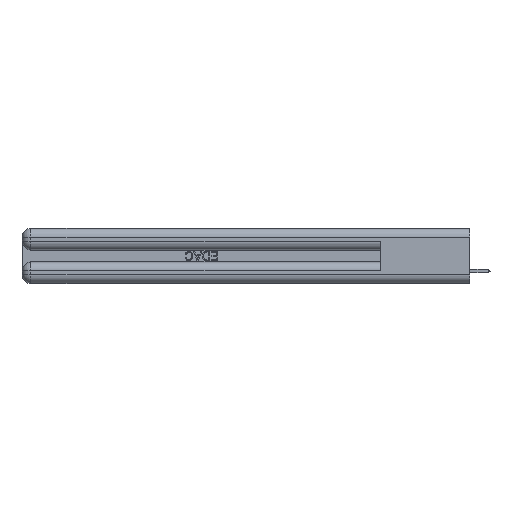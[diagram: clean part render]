
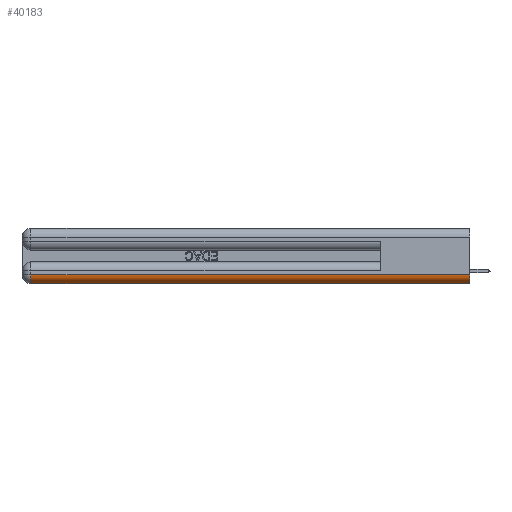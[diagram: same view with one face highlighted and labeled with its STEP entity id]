
A CAD part, left-side view. The second image highlights one B-rep face of the part: STEP entity #40183.
In plain terms, the highlighted cylindrical face has radius 1.524 mm (diameter 3.048 mm), a partial arc.
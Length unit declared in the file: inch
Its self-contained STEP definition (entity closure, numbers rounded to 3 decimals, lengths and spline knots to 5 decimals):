
#938 = DIRECTION ( 'NONE',  ( 0., -1., 0. ) ) ;
#4391 = EDGE_CURVE ( 'NONE', #38778, #20367, #21071, .T. ) ;
#5173 = CARTESIAN_POINT ( 'NONE',  ( 0.06, 0., 0. ) ) ;
#5672 = VECTOR ( 'NONE', #938, 39.37008 ) ;
#6079 = CARTESIAN_POINT ( 'NONE',  ( 0.06, 2.94, 0. ) ) ;
#6116 = LINE ( 'NONE', #17339, #40476 ) ;
#7012 = AXIS2_PLACEMENT_3D ( 'NONE', #14350, #36094, #39672 ) ;
#9419 = DIRECTION ( 'NONE',  ( 0., -1., 0. ) ) ;
#10543 = VERTEX_POINT ( 'NONE', #6079 ) ;
#13378 = EDGE_CURVE ( 'NONE', #28678, #38778, #43937, .T. ) ;
#13647 = ORIENTED_EDGE ( 'NONE', *, *, #13378, .F. ) ;
#14350 = CARTESIAN_POINT ( 'NONE',  ( 0.06, 2.94, 0.06 ) ) ;
#15089 = FACE_OUTER_BOUND ( 'NONE', #19621, .T. ) ;
#17255 = AXIS2_PLACEMENT_3D ( 'NONE', #27853, #9419, #34544 ) ;
#17339 = CARTESIAN_POINT ( 'NONE',  ( 0.06, 3., 0. ) ) ;
#17907 = CYLINDRICAL_SURFACE ( 'NONE', #21600, 0.06 ) ;
#18154 = ORIENTED_EDGE ( 'NONE', *, *, #30021, .F. ) ;
#19589 = CARTESIAN_POINT ( 'NONE',  ( 0., 0., 0.06 ) ) ;
#19608 = CIRCLE ( 'NONE', #7012, 0.06 ) ;
#19621 = EDGE_LOOP ( 'NONE', ( #29744, #13647, #32563, #18154 ) ) ;
#19750 = DIRECTION ( 'NONE',  ( 0., 0., 1. ) ) ;
#20367 = VERTEX_POINT ( 'NONE', #5173 ) ;
#21071 = CIRCLE ( 'NONE', #17255, 0.06 ) ;
#21600 = AXIS2_PLACEMENT_3D ( 'NONE', #34498, #30189, #19750 ) ;
#26704 = CARTESIAN_POINT ( 'NONE',  ( 0., 0., 0.06 ) ) ;
#27853 = CARTESIAN_POINT ( 'NONE',  ( 0.06, 0., 0.06 ) ) ;
#28678 = VERTEX_POINT ( 'NONE', #43455 ) ;
#29744 = ORIENTED_EDGE ( 'NONE', *, *, #4391, .F. ) ;
#30021 = EDGE_CURVE ( 'NONE', #20367, #10543, #6116, .T. ) ;
#30189 = DIRECTION ( 'NONE',  ( 0., 1., 0. ) ) ;
#32563 = ORIENTED_EDGE ( 'NONE', *, *, #44700, .F. ) ;
#34498 = CARTESIAN_POINT ( 'NONE',  ( 0.06, 0., 0.06 ) ) ;
#34544 = DIRECTION ( 'NONE',  ( 0., 0., 1. ) ) ;
#35816 = DIRECTION ( 'NONE',  ( 0., 1., 0. ) ) ;
#36094 = DIRECTION ( 'NONE',  ( 0., 1., 0. ) ) ;
#38778 = VERTEX_POINT ( 'NONE', #19589 ) ;
#39672 = DIRECTION ( 'NONE',  ( 0., 0., 1. ) ) ;
#40183 = ADVANCED_FACE ( 'NONE', ( #15089 ), #17907, .T. ) ;
#40476 = VECTOR ( 'NONE', #35816, 39.37008 ) ;
#43455 = CARTESIAN_POINT ( 'NONE',  ( 0., 2.94, 0.06 ) ) ;
#43937 = LINE ( 'NONE', #26704, #5672 ) ;
#44700 = EDGE_CURVE ( 'NONE', #10543, #28678, #19608, .T. ) ;
